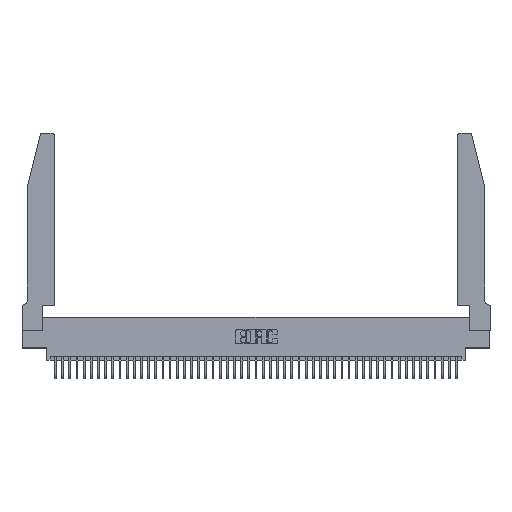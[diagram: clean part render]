
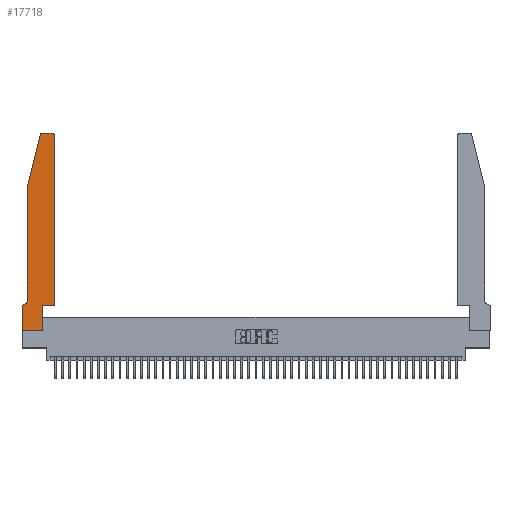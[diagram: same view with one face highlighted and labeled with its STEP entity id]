
A CAD part, top view. The second image highlights one B-rep face of the part: STEP entity #17718.
In plain terms, the highlighted planar face has unit normal (0, 0, 1).
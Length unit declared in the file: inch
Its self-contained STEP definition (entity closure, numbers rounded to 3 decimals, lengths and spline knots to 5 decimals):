
#241 = VERTEX_POINT ( 'NONE', #37135 ) ;
#272 = CIRCLE ( 'NONE', #33591, 0.07 ) ;
#364 = EDGE_CURVE ( 'NONE', #13181, #26968, #35586, .T. ) ;
#1029 = DIRECTION ( 'NONE',  ( 1., 0., 0. ) ) ;
#1469 = FACE_OUTER_BOUND ( 'NONE', #39976, .T. ) ;
#1510 = DIRECTION ( 'NONE',  ( 0., 0., 1. ) ) ;
#2144 = VERTEX_POINT ( 'NONE', #15101 ) ;
#2148 = LINE ( 'NONE', #33944, #29279 ) ;
#2862 = CARTESIAN_POINT ( 'NONE',  ( 0.2865, 0., 0.37 ) ) ;
#2880 = VERTEX_POINT ( 'NONE', #4686 ) ;
#3265 = ORIENTED_EDGE ( 'NONE', *, *, #16960, .T. ) ;
#3542 = CARTESIAN_POINT ( 'NONE',  ( 0.0755, 2., 0.37 ) ) ;
#3672 = EDGE_CURVE ( 'NONE', #26968, #28269, #2148, .T. ) ;
#4404 = VECTOR ( 'NONE', #24409, 39.37008 ) ;
#4495 = EDGE_CURVE ( 'NONE', #41368, #30263, #8567, .T. ) ;
#4686 = CARTESIAN_POINT ( 'NONE',  ( 0.0755, 0.42, 0.37 ) ) ;
#5610 = LINE ( 'NONE', #11030, #31530 ) ;
#5692 = ORIENTED_EDGE ( 'NONE', *, *, #37991, .T. ) ;
#5830 = DIRECTION ( 'NONE',  ( 0., 0., -1. ) ) ;
#6514 = ORIENTED_EDGE ( 'NONE', *, *, #27299, .T. ) ;
#6612 = CARTESIAN_POINT ( 'NONE',  ( 0.2865, 0.35, 0.37 ) ) ;
#6627 = EDGE_CURVE ( 'NONE', #42540, #41368, #22804, .T. ) ;
#6786 = CARTESIAN_POINT ( 'NONE',  ( 0.4205, 2.72, 0.37 ) ) ;
#7471 = VECTOR ( 'NONE', #39287, 39.37008 ) ;
#7724 = ORIENTED_EDGE ( 'NONE', *, *, #26807, .T. ) ;
#7885 = EDGE_CURVE ( 'NONE', #28269, #2144, #36427, .T. ) ;
#8567 = LINE ( 'NONE', #16058, #35581 ) ;
#9204 = ORIENTED_EDGE ( 'NONE', *, *, #364, .T. ) ;
#10311 = DIRECTION ( 'NONE',  ( 1., 0., 0. ) ) ;
#10804 = CARTESIAN_POINT ( 'NONE',  ( 0.4505, 0.35, 0.37 ) ) ;
#11030 = CARTESIAN_POINT ( 'NONE',  ( 0.0755, 0.35, 0.37 ) ) ;
#11117 = ORIENTED_EDGE ( 'NONE', *, *, #6627, .T. ) ;
#12018 = CARTESIAN_POINT ( 'NONE',  ( 0.25487, 2.72718, 0.37 ) ) ;
#12814 = DIRECTION ( 'NONE',  ( 1., 0., 0. ) ) ;
#13181 = VERTEX_POINT ( 'NONE', #2862 ) ;
#13455 = ORIENTED_EDGE ( 'NONE', *, *, #3672, .T. ) ;
#13862 = CARTESIAN_POINT ( 'NONE',  ( 0.284, 2.72, 0.37 ) ) ;
#14280 = ORIENTED_EDGE ( 'NONE', *, *, #24837, .T. ) ;
#14356 = VERTEX_POINT ( 'NONE', #34295 ) ;
#15101 = CARTESIAN_POINT ( 'NONE',  ( 0.4505, 2.72, 0.37 ) ) ;
#15209 = CARTESIAN_POINT ( 'NONE',  ( 0., 0., 0.37 ) ) ;
#15360 = VECTOR ( 'NONE', #1029, 39.37008 ) ;
#16058 = CARTESIAN_POINT ( 'NONE',  ( 0.0755, 2., 0.37 ) ) ;
#16333 = EDGE_CURVE ( 'NONE', #35550, #42540, #30064, .T. ) ;
#16571 = ORIENTED_EDGE ( 'NONE', *, *, #4495, .T. ) ;
#16960 = EDGE_CURVE ( 'NONE', #30263, #2880, #32574, .T. ) ;
#16981 = AXIS2_PLACEMENT_3D ( 'NONE', #6786, #31426, #10311 ) ;
#17396 = DIRECTION ( 'NONE',  ( 1., 0., 0. ) ) ;
#17718 = ADVANCED_FACE ( 'NONE', ( #1469 ), #19216, .T. ) ;
#17801 = EDGE_CURVE ( 'NONE', #14356, #241, #34709, .T. ) ;
#18656 = ORIENTED_EDGE ( 'NONE', *, *, #17801, .T. ) ;
#19216 = PLANE ( 'NONE',  #40237 ) ;
#19582 = VECTOR ( 'NONE', #24623, 39.37008 ) ;
#20714 = VERTEX_POINT ( 'NONE', #42614 ) ;
#20989 = CARTESIAN_POINT ( 'NONE',  ( 0.4505, 0.35, 0.37 ) ) ;
#21493 = CARTESIAN_POINT ( 'NONE',  ( 0.2865, 0.35, 0.37 ) ) ;
#22804 = CIRCLE ( 'NONE', #41086, 0.03 ) ;
#23111 = CARTESIAN_POINT ( 'NONE',  ( 0., 0., 0.37 ) ) ;
#23112 = ORIENTED_EDGE ( 'NONE', *, *, #16333, .T. ) ;
#24409 = DIRECTION ( 'NONE',  ( 0., -1., 0. ) ) ;
#24562 = DIRECTION ( 'NONE',  ( 0., 1., 0. ) ) ;
#24574 = CARTESIAN_POINT ( 'NONE',  ( 0.0755, 2., 0.37 ) ) ;
#24623 = DIRECTION ( 'NONE',  ( -1., 0., 0. ) ) ;
#24761 = LINE ( 'NONE', #15209, #15360 ) ;
#24837 = EDGE_CURVE ( 'NONE', #20714, #14356, #5610, .T. ) ;
#25318 = VECTOR ( 'NONE', #37226, 39.37008 ) ;
#25963 = CARTESIAN_POINT ( 'NONE',  ( 0.4205, 2.75, 0.37 ) ) ;
#26299 = DIRECTION ( 'NONE',  ( 1., 0., 0. ) ) ;
#26670 = DIRECTION ( 'NONE',  ( -0.239, -0.971, 0. ) ) ;
#26807 = EDGE_CURVE ( 'NONE', #2880, #20714, #272, .T. ) ;
#26953 = CARTESIAN_POINT ( 'NONE',  ( 0.0055, 0.42, 0.37 ) ) ;
#26968 = VERTEX_POINT ( 'NONE', #6612 ) ;
#27045 = VECTOR ( 'NONE', #24562, 39.37008 ) ;
#27299 = EDGE_CURVE ( 'NONE', #241, #13181, #24761, .T. ) ;
#28112 = CIRCLE ( 'NONE', #16981, 0.03 ) ;
#28269 = VERTEX_POINT ( 'NONE', #10804 ) ;
#28336 = ORIENTED_EDGE ( 'NONE', *, *, #7885, .T. ) ;
#28584 = DIRECTION ( 'NONE',  ( -1., 0., 0. ) ) ;
#29279 = VECTOR ( 'NONE', #12814, 39.37008 ) ;
#30064 = LINE ( 'NONE', #42139, #19582 ) ;
#30263 = VERTEX_POINT ( 'NONE', #3542 ) ;
#30496 = DIRECTION ( 'NONE',  ( -1., 0., 0. ) ) ;
#31426 = DIRECTION ( 'NONE',  ( 0., 0., 1. ) ) ;
#31530 = VECTOR ( 'NONE', #28584, 39.37008 ) ;
#32574 = LINE ( 'NONE', #24574, #4404 ) ;
#33591 = AXIS2_PLACEMENT_3D ( 'NONE', #26953, #5830, #30496 ) ;
#33944 = CARTESIAN_POINT ( 'NONE',  ( 0.4505, 0.35, 0.37 ) ) ;
#34295 = CARTESIAN_POINT ( 'NONE',  ( 0., 0.35, 0.37 ) ) ;
#34709 = LINE ( 'NONE', #23111, #25318 ) ;
#35550 = VERTEX_POINT ( 'NONE', #25963 ) ;
#35581 = VECTOR ( 'NONE', #26670, 39.37008 ) ;
#35586 = LINE ( 'NONE', #21493, #7471 ) ;
#36427 = LINE ( 'NONE', #20989, #27045 ) ;
#37135 = CARTESIAN_POINT ( 'NONE',  ( 0., 0., 0.37 ) ) ;
#37226 = DIRECTION ( 'NONE',  ( 0., -1., 0. ) ) ;
#37991 = EDGE_CURVE ( 'NONE', #2144, #35550, #28112, .T. ) ;
#38551 = DIRECTION ( 'NONE',  ( 0., 0., 1. ) ) ;
#39287 = DIRECTION ( 'NONE',  ( 0., 1., 0. ) ) ;
#39976 = EDGE_LOOP ( 'NONE', ( #23112, #11117, #16571, #3265, #7724, #14280, #18656, #6514, #9204, #13455, #28336, #5692 ) ) ;
#40237 = AXIS2_PLACEMENT_3D ( 'NONE', #43863, #1510, #26299 ) ;
#41086 = AXIS2_PLACEMENT_3D ( 'NONE', #13862, #38551, #17396 ) ;
#41368 = VERTEX_POINT ( 'NONE', #12018 ) ;
#42139 = CARTESIAN_POINT ( 'NONE',  ( 0.2605, 2.75, 0.37 ) ) ;
#42540 = VERTEX_POINT ( 'NONE', #42874 ) ;
#42614 = CARTESIAN_POINT ( 'NONE',  ( 0.0055, 0.35, 0.37 ) ) ;
#42874 = CARTESIAN_POINT ( 'NONE',  ( 0.284, 2.75, 0.37 ) ) ;
#43863 = CARTESIAN_POINT ( 'NONE',  ( 0., 0.35, 0.37 ) ) ;
